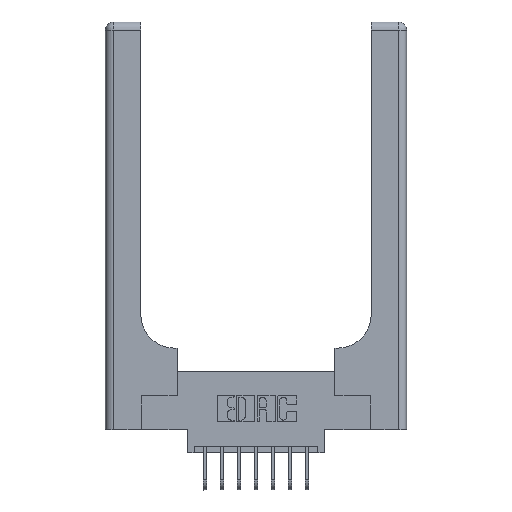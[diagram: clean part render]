
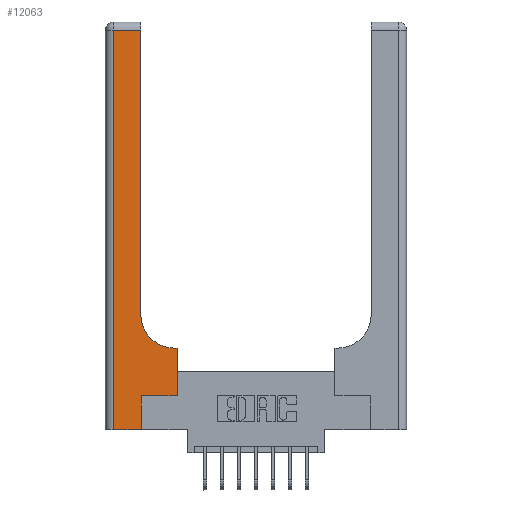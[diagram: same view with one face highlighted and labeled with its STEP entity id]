
A CAD part, top view. The second image highlights one B-rep face of the part: STEP entity #12063.
In plain terms, the highlighted planar face has unit normal (0, 0, 1).
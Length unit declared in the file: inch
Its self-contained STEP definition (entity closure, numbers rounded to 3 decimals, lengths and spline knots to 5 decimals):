
#74 = ORIENTED_EDGE ( 'NONE', *, *, #3626, .T. ) ;
#114 = PLANE ( 'NONE',  #8163 ) ;
#142 = DIRECTION ( 'NONE',  ( 1., 0., 0. ) ) ;
#354 = EDGE_CURVE ( 'NONE', #9902, #5010, #7206, .T. ) ;
#359 = ORIENTED_EDGE ( 'NONE', *, *, #13942, .T. ) ;
#600 = ORIENTED_EDGE ( 'NONE', *, *, #15419, .T. ) ;
#680 = DIRECTION ( 'NONE',  ( 0., 1., 0. ) ) ;
#1452 = EDGE_CURVE ( 'NONE', #13436, #9902, #8546, .T. ) ;
#1904 = VERTEX_POINT ( 'NONE', #5279 ) ;
#1976 = VERTEX_POINT ( 'NONE', #6586 ) ;
#2150 = DIRECTION ( 'NONE',  ( 1., 0., 0. ) ) ;
#2904 = EDGE_CURVE ( 'NONE', #5010, #1904, #12321, .T. ) ;
#3115 = VERTEX_POINT ( 'NONE', #12013 ) ;
#3495 = VECTOR ( 'NONE', #5948, 39.37008 ) ;
#3536 = ORIENTED_EDGE ( 'NONE', *, *, #354, .T. ) ;
#3591 = EDGE_CURVE ( 'NONE', #13144, #1976, #13028, .T. ) ;
#3626 = EDGE_CURVE ( 'NONE', #8801, #13436, #4575, .T. ) ;
#3883 = ORIENTED_EDGE ( 'NONE', *, *, #7270, .T. ) ;
#4291 = DIRECTION ( 'NONE',  ( 0., 0., -1. ) ) ;
#4575 = LINE ( 'NONE', #12544, #14431 ) ;
#5010 = VERTEX_POINT ( 'NONE', #8837 ) ;
#5268 = CARTESIAN_POINT ( 'NONE',  ( 0., 2.94, 0.37 ) ) ;
#5279 = CARTESIAN_POINT ( 'NONE',  ( 0.528, 0.25, 0.37 ) ) ;
#5948 = DIRECTION ( 'NONE',  ( 0., 1., 0. ) ) ;
#6063 = DIRECTION ( 'NONE',  ( 1., 0., 0. ) ) ;
#6446 = LINE ( 'NONE', #7927, #10794 ) ;
#6586 = CARTESIAN_POINT ( 'NONE',  ( 0.26, 2.94, 0.37 ) ) ;
#6923 = DIRECTION ( 'NONE',  ( 0., 1., 0. ) ) ;
#7051 = ORIENTED_EDGE ( 'NONE', *, *, #10771, .T. ) ;
#7201 = CARTESIAN_POINT ( 'NONE',  ( 0.51, 0.85, 0.37 ) ) ;
#7206 = LINE ( 'NONE', #14850, #3495 ) ;
#7270 = EDGE_CURVE ( 'NONE', #8904, #3115, #14703, .T. ) ;
#7927 = CARTESIAN_POINT ( 'NONE',  ( 0.528, 0.25, 0.37 ) ) ;
#8163 = AXIS2_PLACEMENT_3D ( 'NONE', #13813, #4291, #13672 ) ;
#8469 = VECTOR ( 'NONE', #680, 39.37008 ) ;
#8521 = CARTESIAN_POINT ( 'NONE',  ( 0.528, 0.6, 0.37 ) ) ;
#8546 = LINE ( 'NONE', #14787, #14932 ) ;
#8801 = VERTEX_POINT ( 'NONE', #15649 ) ;
#8837 = CARTESIAN_POINT ( 'NONE',  ( 0.265, 0.25, 0.37 ) ) ;
#8904 = VERTEX_POINT ( 'NONE', #8521 ) ;
#9902 = VERTEX_POINT ( 'NONE', #15626 ) ;
#10032 = ORIENTED_EDGE ( 'NONE', *, *, #3591, .T. ) ;
#10325 = VECTOR ( 'NONE', #142, 39.37008 ) ;
#10771 = EDGE_CURVE ( 'NONE', #1904, #8904, #6446, .T. ) ;
#10794 = VECTOR ( 'NONE', #6923, 39.37008 ) ;
#10835 = ORIENTED_EDGE ( 'NONE', *, *, #1452, .T. ) ;
#11436 = CARTESIAN_POINT ( 'NONE',  ( 0.06, 0., 0.37 ) ) ;
#11689 = CARTESIAN_POINT ( 'NONE',  ( 0.265, 0.25, 0.37 ) ) ;
#12009 = VECTOR ( 'NONE', #14119, 39.37008 ) ;
#12013 = CARTESIAN_POINT ( 'NONE',  ( 0.51, 0.6, 0.37 ) ) ;
#12063 = ADVANCED_FACE ( 'NONE', ( #16346 ), #114, .F. ) ;
#12321 = LINE ( 'NONE', #11689, #10325 ) ;
#12352 = CARTESIAN_POINT ( 'NONE',  ( 0.26, 0.6, 0.37 ) ) ;
#12473 = VECTOR ( 'NONE', #13652, 39.37008 ) ;
#12544 = CARTESIAN_POINT ( 'NONE',  ( 0.06, 3., 0.37 ) ) ;
#13028 = LINE ( 'NONE', #14594, #8469 ) ;
#13144 = VERTEX_POINT ( 'NONE', #15364 ) ;
#13436 = VERTEX_POINT ( 'NONE', #11436 ) ;
#13652 = DIRECTION ( 'NONE',  ( -1., 0., 0. ) ) ;
#13672 = DIRECTION ( 'NONE',  ( -1., 0., 0. ) ) ;
#13813 = CARTESIAN_POINT ( 'NONE',  ( 0., 3., 0.37 ) ) ;
#13846 = AXIS2_PLACEMENT_3D ( 'NONE', #7201, #16042, #6063 ) ;
#13942 = EDGE_CURVE ( 'NONE', #1976, #8801, #14005, .T. ) ;
#14005 = LINE ( 'NONE', #5268, #12009 ) ;
#14092 = EDGE_LOOP ( 'NONE', ( #10032, #359, #74, #10835, #3536, #15783, #7051, #3883, #600 ) ) ;
#14119 = DIRECTION ( 'NONE',  ( -1., 0., 0. ) ) ;
#14431 = VECTOR ( 'NONE', #15914, 39.37008 ) ;
#14594 = CARTESIAN_POINT ( 'NONE',  ( 0.26, 3., 0.37 ) ) ;
#14703 = LINE ( 'NONE', #12352, #12473 ) ;
#14787 = CARTESIAN_POINT ( 'NONE',  ( 0., 0., 0.37 ) ) ;
#14850 = CARTESIAN_POINT ( 'NONE',  ( 0.265, 0., 0.37 ) ) ;
#14875 = CIRCLE ( 'NONE', #13846, 0.25 ) ;
#14932 = VECTOR ( 'NONE', #2150, 39.37008 ) ;
#15364 = CARTESIAN_POINT ( 'NONE',  ( 0.26, 0.85, 0.37 ) ) ;
#15419 = EDGE_CURVE ( 'NONE', #3115, #13144, #14875, .T. ) ;
#15626 = CARTESIAN_POINT ( 'NONE',  ( 0.265, 0., 0.37 ) ) ;
#15649 = CARTESIAN_POINT ( 'NONE',  ( 0.06, 2.94, 0.37 ) ) ;
#15783 = ORIENTED_EDGE ( 'NONE', *, *, #2904, .T. ) ;
#15914 = DIRECTION ( 'NONE',  ( 0., -1., 0. ) ) ;
#16042 = DIRECTION ( 'NONE',  ( 0., 0., -1. ) ) ;
#16346 = FACE_OUTER_BOUND ( 'NONE', #14092, .T. ) ;
